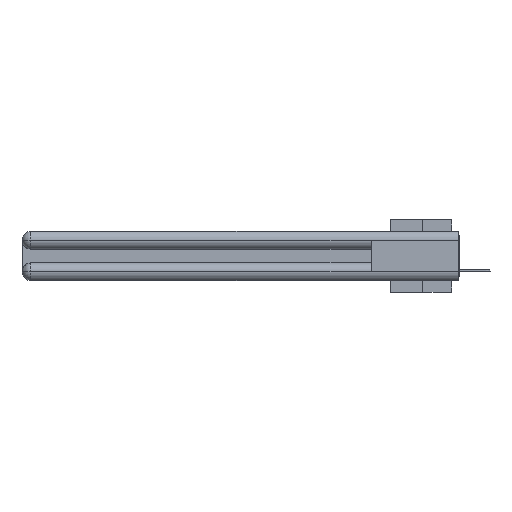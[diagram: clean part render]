
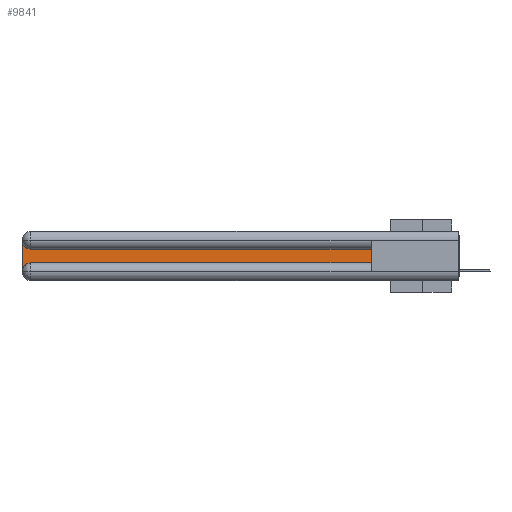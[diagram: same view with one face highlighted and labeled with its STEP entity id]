
A CAD part, left-side view. The second image highlights one B-rep face of the part: STEP entity #9841.
In plain terms, the highlighted planar face has unit normal (-1, 0, 0).
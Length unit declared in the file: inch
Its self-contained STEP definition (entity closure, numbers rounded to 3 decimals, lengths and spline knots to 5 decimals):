
#24 = AXIS2_PLACEMENT_3D ( 'NONE', #37175, #19573, #26236 ) ;
#1614 = PLANE ( 'NONE',  #6531 ) ;
#2293 = VERTEX_POINT ( 'NONE', #23452 ) ;
#2538 = DIRECTION ( 'NONE',  ( 0., -1., 0. ) ) ;
#2699 = DIRECTION ( 'NONE',  ( 0., 0., 1. ) ) ;
#2770 = EDGE_CURVE ( 'NONE', #12916, #23059, #23081, .T. ) ;
#2791 = VECTOR ( 'NONE', #27520, 39.37008 ) ;
#3180 = CARTESIAN_POINT ( 'NONE',  ( 0.075, 2.94, -0.2175 ) ) ;
#4908 = CARTESIAN_POINT ( 'NONE',  ( 0.075, 3., -0.1225 ) ) ;
#4993 = EDGE_CURVE ( 'NONE', #23059, #2293, #32697, .T. ) ;
#5508 = CARTESIAN_POINT ( 'NONE',  ( 0.075, 2.94, -0.0625 ) ) ;
#5971 = EDGE_CURVE ( 'NONE', #32633, #12916, #10580, .T. ) ;
#6531 = AXIS2_PLACEMENT_3D ( 'NONE', #4908, #28227, #22053 ) ;
#8484 = LINE ( 'NONE', #37396, #34585 ) ;
#9841 = ADVANCED_FACE ( 'NONE', ( #28619 ), #1614, .F. ) ;
#9864 = CARTESIAN_POINT ( 'NONE',  ( 0.075, 3., -0.2175 ) ) ;
#10580 = LINE ( 'NONE', #33724, #2791 ) ;
#12868 = VERTEX_POINT ( 'NONE', #3180 ) ;
#12916 = VERTEX_POINT ( 'NONE', #26708 ) ;
#13870 = ORIENTED_EDGE ( 'NONE', *, *, #14427, .T. ) ;
#14427 = EDGE_CURVE ( 'NONE', #12868, #33455, #8484, .T. ) ;
#14449 = ORIENTED_EDGE ( 'NONE', *, *, #34082, .T. ) ;
#17159 = CARTESIAN_POINT ( 'NONE',  ( 0.075, 0.6, -0.2175 ) ) ;
#17602 = CIRCLE ( 'NONE', #24, 0.06 ) ;
#19573 = DIRECTION ( 'NONE',  ( 1., 0., 0. ) ) ;
#19803 = VECTOR ( 'NONE', #36273, 39.37008 ) ;
#20471 = ORIENTED_EDGE ( 'NONE', *, *, #4993, .T. ) ;
#21626 = ORIENTED_EDGE ( 'NONE', *, *, #2770, .T. ) ;
#21893 = EDGE_LOOP ( 'NONE', ( #35210, #21626, #20471, #14449, #13870, #28079 ) ) ;
#22053 = DIRECTION ( 'NONE',  ( 0., 0., -1. ) ) ;
#23059 = VERTEX_POINT ( 'NONE', #31968 ) ;
#23081 = CIRCLE ( 'NONE', #32432, 0.06 ) ;
#23452 = CARTESIAN_POINT ( 'NONE',  ( 0.075, 3., -0.2775 ) ) ;
#23965 = VECTOR ( 'NONE', #2699, 39.37008 ) ;
#26236 = DIRECTION ( 'NONE',  ( 0., 0., -1. ) ) ;
#26708 = CARTESIAN_POINT ( 'NONE',  ( 0.075, 2.94, -0.1225 ) ) ;
#27520 = DIRECTION ( 'NONE',  ( 0., 1., 0. ) ) ;
#28079 = ORIENTED_EDGE ( 'NONE', *, *, #31041, .T. ) ;
#28227 = DIRECTION ( 'NONE',  ( 1., 0., 0. ) ) ;
#28619 = FACE_OUTER_BOUND ( 'NONE', #21893, .T. ) ;
#30721 = CARTESIAN_POINT ( 'NONE',  ( 0.075, 0.6, -0.1225 ) ) ;
#31041 = EDGE_CURVE ( 'NONE', #33455, #32633, #37767, .T. ) ;
#31797 = DIRECTION ( 'NONE',  ( 0., 0., -1. ) ) ;
#31968 = CARTESIAN_POINT ( 'NONE',  ( 0.075, 3., -0.0625 ) ) ;
#32432 = AXIS2_PLACEMENT_3D ( 'NONE', #5508, #37941, #31797 ) ;
#32633 = VERTEX_POINT ( 'NONE', #30721 ) ;
#32697 = LINE ( 'NONE', #9864, #19803 ) ;
#33455 = VERTEX_POINT ( 'NONE', #34909 ) ;
#33724 = CARTESIAN_POINT ( 'NONE',  ( 0.075, 0.6, -0.1225 ) ) ;
#34082 = EDGE_CURVE ( 'NONE', #2293, #12868, #17602, .T. ) ;
#34585 = VECTOR ( 'NONE', #2538, 39.37008 ) ;
#34909 = CARTESIAN_POINT ( 'NONE',  ( 0.075, 0.6, -0.2175 ) ) ;
#35210 = ORIENTED_EDGE ( 'NONE', *, *, #5971, .T. ) ;
#36273 = DIRECTION ( 'NONE',  ( 0., 0., -1. ) ) ;
#37175 = CARTESIAN_POINT ( 'NONE',  ( 0.075, 2.94, -0.2775 ) ) ;
#37396 = CARTESIAN_POINT ( 'NONE',  ( 0.075, 0.6, -0.2175 ) ) ;
#37767 = LINE ( 'NONE', #17159, #23965 ) ;
#37941 = DIRECTION ( 'NONE',  ( 1., 0., 0. ) ) ;
